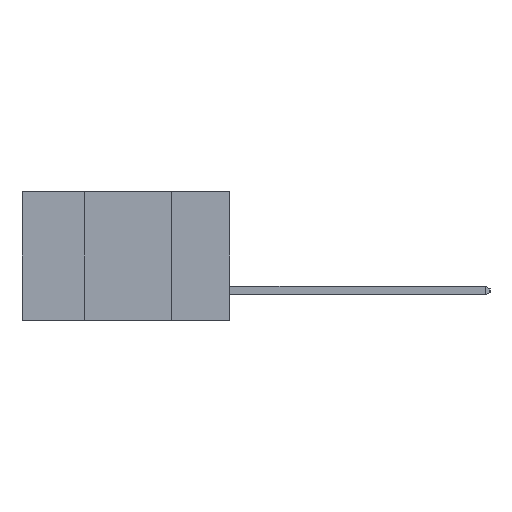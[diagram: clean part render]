
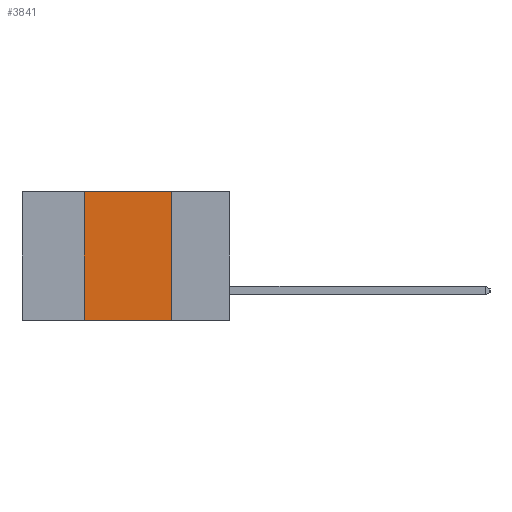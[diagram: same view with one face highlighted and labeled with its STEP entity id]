
A CAD part, left-side view. The second image highlights one B-rep face of the part: STEP entity #3841.
In plain terms, the highlighted planar face has unit normal (-1, 0, 0).
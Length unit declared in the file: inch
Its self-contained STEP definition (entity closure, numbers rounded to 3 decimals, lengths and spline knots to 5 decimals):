
#673 = VERTEX_POINT ( 'NONE', #11300 ) ;
#771 = AXIS2_PLACEMENT_3D ( 'NONE', #13728, #13670, #13659 ) ;
#1516 = ORIENTED_EDGE ( 'NONE', *, *, #17141, .T. ) ;
#2188 = LINE ( 'NONE', #7018, #12931 ) ;
#2380 = LINE ( 'NONE', #6610, #10029 ) ;
#2492 = CARTESIAN_POINT ( 'NONE',  ( 0., 0.42, -0.37 ) ) ;
#3693 = ORIENTED_EDGE ( 'NONE', *, *, #8186, .F. ) ;
#3841 = ADVANCED_FACE ( 'NONE', ( #15428 ), #13804, .F. ) ;
#5070 = VECTOR ( 'NONE', #16603, 39.37008 ) ;
#5791 = CARTESIAN_POINT ( 'NONE',  ( 0., 0.17, 0. ) ) ;
#6610 = CARTESIAN_POINT ( 'NONE',  ( 0., 0.42, -0.37 ) ) ;
#7018 = CARTESIAN_POINT ( 'NONE',  ( 0., 0.6, -0.37 ) ) ;
#7109 = CARTESIAN_POINT ( 'NONE',  ( 0., 0.17, -0.37 ) ) ;
#8121 = DIRECTION ( 'NONE',  ( 0., 0., 1. ) ) ;
#8186 = EDGE_CURVE ( 'NONE', #18879, #18335, #14320, .T. ) ;
#8188 = ORIENTED_EDGE ( 'NONE', *, *, #16724, .F. ) ;
#8558 = DIRECTION ( 'NONE',  ( 0., -1., 0. ) ) ;
#9034 = CARTESIAN_POINT ( 'NONE',  ( 0., 0.6, 0. ) ) ;
#9588 = LINE ( 'NONE', #9034, #5070 ) ;
#10029 = VECTOR ( 'NONE', #8121, 39.37008 ) ;
#10275 = VECTOR ( 'NONE', #18688, 39.37008 ) ;
#11152 = CARTESIAN_POINT ( 'NONE',  ( 0., 0.17, -0.37 ) ) ;
#11300 = CARTESIAN_POINT ( 'NONE',  ( 0., 0.42, 0. ) ) ;
#12931 = VECTOR ( 'NONE', #8558, 39.37008 ) ;
#13659 = DIRECTION ( 'NONE',  ( 0., 0., -1. ) ) ;
#13670 = DIRECTION ( 'NONE',  ( 1., 0., 0. ) ) ;
#13728 = CARTESIAN_POINT ( 'NONE',  ( 0., 0.6, 0. ) ) ;
#13804 = PLANE ( 'NONE',  #771 ) ;
#14320 = LINE ( 'NONE', #11152, #10275 ) ;
#15143 = VERTEX_POINT ( 'NONE', #2492 ) ;
#15428 = FACE_OUTER_BOUND ( 'NONE', #15608, .T. ) ;
#15608 = EDGE_LOOP ( 'NONE', ( #3693, #8188, #16759, #1516 ) ) ;
#16603 = DIRECTION ( 'NONE',  ( 0., -1., 0. ) ) ;
#16724 = EDGE_CURVE ( 'NONE', #673, #18879, #9588, .T. ) ;
#16759 = ORIENTED_EDGE ( 'NONE', *, *, #18125, .F. ) ;
#17141 = EDGE_CURVE ( 'NONE', #15143, #18335, #2188, .T. ) ;
#18125 = EDGE_CURVE ( 'NONE', #15143, #673, #2380, .T. ) ;
#18335 = VERTEX_POINT ( 'NONE', #7109 ) ;
#18688 = DIRECTION ( 'NONE',  ( 0., 0., -1. ) ) ;
#18879 = VERTEX_POINT ( 'NONE', #5791 ) ;
